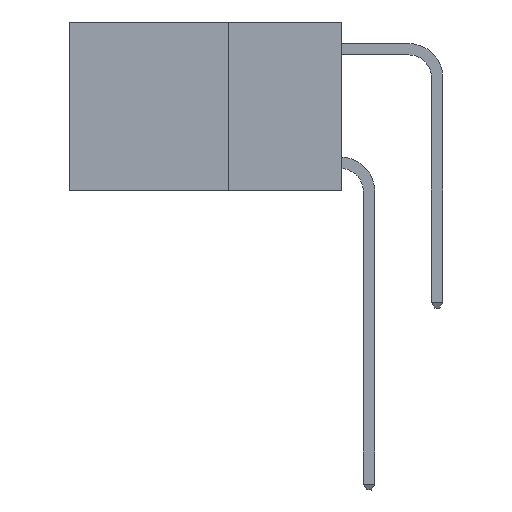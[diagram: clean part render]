
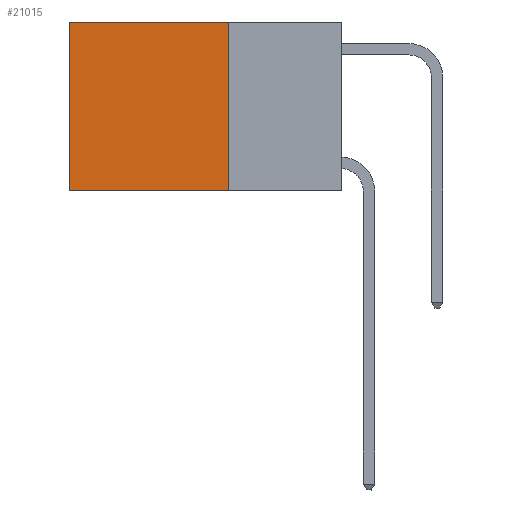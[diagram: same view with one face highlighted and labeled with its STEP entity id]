
A CAD part, left-side view. The second image highlights one B-rep face of the part: STEP entity #21015.
In plain terms, the highlighted planar face has unit normal (-1, 0, 0).
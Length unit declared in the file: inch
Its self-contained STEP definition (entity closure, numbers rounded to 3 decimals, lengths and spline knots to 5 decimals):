
#67 = PLANE ( 'NONE',  #20969 ) ;
#456 = DIRECTION ( 'NONE',  ( 0., 1., 0. ) ) ;
#638 = LINE ( 'NONE', #6634, #7923 ) ;
#1721 = CARTESIAN_POINT ( 'NONE',  ( 0.2625, 0.25, 0. ) ) ;
#2103 = EDGE_CURVE ( 'NONE', #5903, #23855, #12244, .T. ) ;
#3274 = VERTEX_POINT ( 'NONE', #6983 ) ;
#3730 = VECTOR ( 'NONE', #13973, 39.37008 ) ;
#3806 = DIRECTION ( 'NONE',  ( 0., 0., -1. ) ) ;
#5221 = LINE ( 'NONE', #21146, #7921 ) ;
#5705 = VERTEX_POINT ( 'NONE', #1721 ) ;
#5903 = VERTEX_POINT ( 'NONE', #14691 ) ;
#6634 = CARTESIAN_POINT ( 'NONE',  ( 0.2625, 0.6, 0. ) ) ;
#6983 = CARTESIAN_POINT ( 'NONE',  ( 0.2625, 0.6, 0. ) ) ;
#7921 = VECTOR ( 'NONE', #15169, 39.37008 ) ;
#7923 = VECTOR ( 'NONE', #22550, 39.37008 ) ;
#9573 = EDGE_LOOP ( 'NONE', ( #20585, #21948, #19600, #12772 ) ) ;
#12244 = LINE ( 'NONE', #24229, #3730 ) ;
#12772 = ORIENTED_EDGE ( 'NONE', *, *, #16337, .T. ) ;
#13973 = DIRECTION ( 'NONE',  ( 0., 1., 0. ) ) ;
#14138 = CARTESIAN_POINT ( 'NONE',  ( 0.2625, 0.25, 0. ) ) ;
#14285 = CARTESIAN_POINT ( 'NONE',  ( 0.2625, 0.6, -0.37 ) ) ;
#14691 = CARTESIAN_POINT ( 'NONE',  ( 0.2625, 0.25, -0.37 ) ) ;
#15169 = DIRECTION ( 'NONE',  ( 0., 0., -1. ) ) ;
#16337 = EDGE_CURVE ( 'NONE', #5705, #3274, #18643, .T. ) ;
#18643 = LINE ( 'NONE', #20374, #24288 ) ;
#19600 = ORIENTED_EDGE ( 'NONE', *, *, #23233, .F. ) ;
#20374 = CARTESIAN_POINT ( 'NONE',  ( 0.2625, 0.25, 0. ) ) ;
#20585 = ORIENTED_EDGE ( 'NONE', *, *, #25803, .T. ) ;
#20969 = AXIS2_PLACEMENT_3D ( 'NONE', #14138, #24135, #3806 ) ;
#21015 = ADVANCED_FACE ( 'NONE', ( #25740 ), #67, .F. ) ;
#21146 = CARTESIAN_POINT ( 'NONE',  ( 0.2625, 0.25, 0. ) ) ;
#21948 = ORIENTED_EDGE ( 'NONE', *, *, #2103, .F. ) ;
#22550 = DIRECTION ( 'NONE',  ( 0., 0., -1. ) ) ;
#23233 = EDGE_CURVE ( 'NONE', #5705, #5903, #5221, .T. ) ;
#23855 = VERTEX_POINT ( 'NONE', #14285 ) ;
#24135 = DIRECTION ( 'NONE',  ( 1., 0., 0. ) ) ;
#24229 = CARTESIAN_POINT ( 'NONE',  ( 0.2625, 0.25, -0.37 ) ) ;
#24288 = VECTOR ( 'NONE', #456, 39.37008 ) ;
#25740 = FACE_OUTER_BOUND ( 'NONE', #9573, .T. ) ;
#25803 = EDGE_CURVE ( 'NONE', #3274, #23855, #638, .T. ) ;
